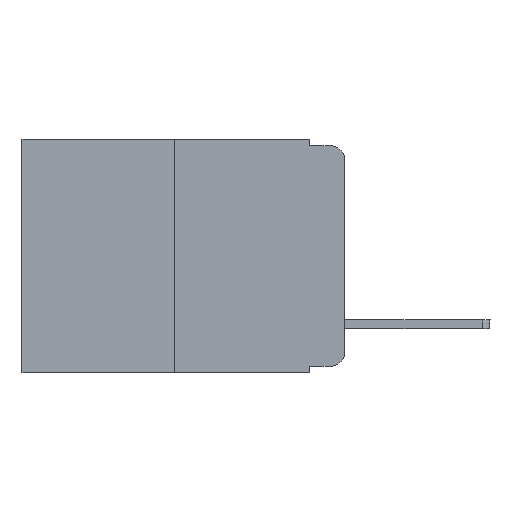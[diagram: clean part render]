
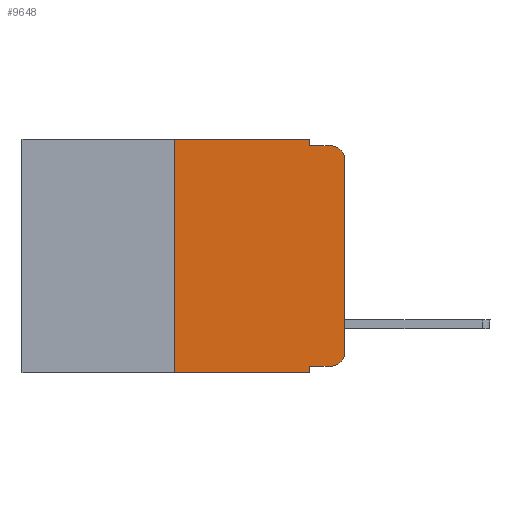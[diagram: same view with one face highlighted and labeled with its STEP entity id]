
A CAD part, left-side view. The second image highlights one B-rep face of the part: STEP entity #9648.
In plain terms, the highlighted planar face has unit normal (-1, 0, 0).
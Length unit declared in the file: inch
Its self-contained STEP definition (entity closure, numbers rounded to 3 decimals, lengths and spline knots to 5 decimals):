
#124 = CARTESIAN_POINT ( 'NONE',  ( 0., 0., -0.313 ) ) ;
#244 = CARTESIAN_POINT ( 'NONE',  ( 0., 0.02, -0.03 ) ) ;
#309 = VERTEX_POINT ( 'NONE', #10297 ) ;
#457 = EDGE_CURVE ( 'NONE', #13211, #309, #10844, .T. ) ;
#489 = LINE ( 'NONE', #7802, #2641 ) ;
#513 = CARTESIAN_POINT ( 'NONE',  ( 0., 0.051, -0.01 ) ) ;
#597 = EDGE_CURVE ( 'NONE', #13211, #7160, #13283, .T. ) ;
#860 = CARTESIAN_POINT ( 'NONE',  ( 0., 0.02, -0.01 ) ) ;
#959 = VECTOR ( 'NONE', #5321, 39.37008 ) ;
#1046 = EDGE_CURVE ( 'NONE', #6598, #12719, #2630, .T. ) ;
#1496 = CARTESIAN_POINT ( 'NONE',  ( 0., 0., 0. ) ) ;
#1751 = LINE ( 'NONE', #15032, #9941 ) ;
#2377 = LINE ( 'NONE', #13235, #959 ) ;
#2577 = CARTESIAN_POINT ( 'NONE',  ( 0., 0.051, -0.333 ) ) ;
#2630 = CIRCLE ( 'NONE', #5128, 0.02 ) ;
#2637 = DIRECTION ( 'NONE',  ( -1., 0., 0. ) ) ;
#2641 = VECTOR ( 'NONE', #2808, 39.37008 ) ;
#2808 = DIRECTION ( 'NONE',  ( 0., 0., 1. ) ) ;
#3148 = DIRECTION ( 'NONE',  ( 1., 0., 0. ) ) ;
#3225 = CIRCLE ( 'NONE', #9435, 0.02 ) ;
#3237 = CARTESIAN_POINT ( 'NONE',  ( 0., 0.051, 0. ) ) ;
#3247 = ORIENTED_EDGE ( 'NONE', *, *, #1046, .T. ) ;
#4075 = PLANE ( 'NONE',  #11360 ) ;
#4367 = DIRECTION ( 'NONE',  ( -1., 0., 0. ) ) ;
#4418 = DIRECTION ( 'NONE',  ( 0., 0., -1. ) ) ;
#4558 = ORIENTED_EDGE ( 'NONE', *, *, #597, .T. ) ;
#4846 = ORIENTED_EDGE ( 'NONE', *, *, #13310, .F. ) ;
#4979 = ORIENTED_EDGE ( 'NONE', *, *, #10083, .F. ) ;
#5128 = AXIS2_PLACEMENT_3D ( 'NONE', #244, #2637, #6245 ) ;
#5206 = ORIENTED_EDGE ( 'NONE', *, *, #10003, .T. ) ;
#5321 = DIRECTION ( 'NONE',  ( 0., -1., 0. ) ) ;
#6245 = DIRECTION ( 'NONE',  ( 0., 0., -1. ) ) ;
#6386 = EDGE_CURVE ( 'NONE', #14319, #11759, #12728, .T. ) ;
#6395 = CARTESIAN_POINT ( 'NONE',  ( 0., 0., -0.03 ) ) ;
#6598 = VERTEX_POINT ( 'NONE', #6395 ) ;
#6616 = CARTESIAN_POINT ( 'NONE',  ( 0., 0.25, 0. ) ) ;
#6806 = DIRECTION ( 'NONE',  ( 0., -1., 0. ) ) ;
#7160 = VERTEX_POINT ( 'NONE', #7847 ) ;
#7196 = EDGE_CURVE ( 'NONE', #11759, #10997, #14890, .T. ) ;
#7591 = FACE_OUTER_BOUND ( 'NONE', #10200, .T. ) ;
#7802 = CARTESIAN_POINT ( 'NONE',  ( 0., 0.25, 0. ) ) ;
#7847 = CARTESIAN_POINT ( 'NONE',  ( 0., 0.02, -0.333 ) ) ;
#7875 = CARTESIAN_POINT ( 'NONE',  ( 0., 0.02, -0.313 ) ) ;
#8741 = DIRECTION ( 'NONE',  ( 0., -1., 0. ) ) ;
#9435 = AXIS2_PLACEMENT_3D ( 'NONE', #7875, #4367, #15144 ) ;
#9567 = VECTOR ( 'NONE', #4418, 39.37008 ) ;
#9648 = ADVANCED_FACE ( 'NONE', ( #7591 ), #4075, .F. ) ;
#9941 = VECTOR ( 'NONE', #11351, 39.37008 ) ;
#10003 = EDGE_CURVE ( 'NONE', #11485, #6598, #13209, .T. ) ;
#10083 = EDGE_CURVE ( 'NONE', #11292, #14319, #489, .T. ) ;
#10152 = DIRECTION ( 'NONE',  ( 0., 0., -1. ) ) ;
#10200 = EDGE_LOOP ( 'NONE', ( #5206, #3247, #4846, #13097, #14035, #4979, #12467, #13558, #4558, #13057 ) ) ;
#10297 = CARTESIAN_POINT ( 'NONE',  ( 0., 0.051, -0.343 ) ) ;
#10403 = VECTOR ( 'NONE', #11717, 39.37008 ) ;
#10844 = LINE ( 'NONE', #12887, #10403 ) ;
#10997 = VERTEX_POINT ( 'NONE', #513 ) ;
#11292 = VERTEX_POINT ( 'NONE', #14912 ) ;
#11351 = DIRECTION ( 'NONE',  ( 0., -1., 0. ) ) ;
#11360 = AXIS2_PLACEMENT_3D ( 'NONE', #14784, #3148, #10152 ) ;
#11485 = VERTEX_POINT ( 'NONE', #124 ) ;
#11593 = CARTESIAN_POINT ( 'NONE',  ( 0., 0.051, -0.333 ) ) ;
#11717 = DIRECTION ( 'NONE',  ( 0., 0., -1. ) ) ;
#11759 = VERTEX_POINT ( 'NONE', #3237 ) ;
#11945 = DIRECTION ( 'NONE',  ( 0., 0., 1. ) ) ;
#12368 = VECTOR ( 'NONE', #11945, 39.37008 ) ;
#12467 = ORIENTED_EDGE ( 'NONE', *, *, #14792, .T. ) ;
#12719 = VERTEX_POINT ( 'NONE', #860 ) ;
#12728 = LINE ( 'NONE', #13983, #14267 ) ;
#12887 = CARTESIAN_POINT ( 'NONE',  ( 0., 0.051, 0. ) ) ;
#13057 = ORIENTED_EDGE ( 'NONE', *, *, #13857, .T. ) ;
#13078 = VECTOR ( 'NONE', #8741, 39.37008 ) ;
#13097 = ORIENTED_EDGE ( 'NONE', *, *, #7196, .F. ) ;
#13209 = LINE ( 'NONE', #1496, #12368 ) ;
#13211 = VERTEX_POINT ( 'NONE', #11593 ) ;
#13235 = CARTESIAN_POINT ( 'NONE',  ( 0., 0.051, -0.01 ) ) ;
#13283 = LINE ( 'NONE', #2577, #13078 ) ;
#13310 = EDGE_CURVE ( 'NONE', #10997, #12719, #2377, .T. ) ;
#13558 = ORIENTED_EDGE ( 'NONE', *, *, #457, .F. ) ;
#13711 = CARTESIAN_POINT ( 'NONE',  ( 0., 0.051, 0. ) ) ;
#13857 = EDGE_CURVE ( 'NONE', #7160, #11485, #3225, .T. ) ;
#13983 = CARTESIAN_POINT ( 'NONE',  ( 0., 0.473, 0. ) ) ;
#14035 = ORIENTED_EDGE ( 'NONE', *, *, #6386, .F. ) ;
#14267 = VECTOR ( 'NONE', #6806, 39.37008 ) ;
#14319 = VERTEX_POINT ( 'NONE', #6616 ) ;
#14784 = CARTESIAN_POINT ( 'NONE',  ( 0., 0.473, 0. ) ) ;
#14792 = EDGE_CURVE ( 'NONE', #11292, #309, #1751, .T. ) ;
#14890 = LINE ( 'NONE', #13711, #9567 ) ;
#14912 = CARTESIAN_POINT ( 'NONE',  ( 0., 0.25, -0.343 ) ) ;
#15032 = CARTESIAN_POINT ( 'NONE',  ( 0., 0.473, -0.343 ) ) ;
#15144 = DIRECTION ( 'NONE',  ( 0., 0., -1. ) ) ;
